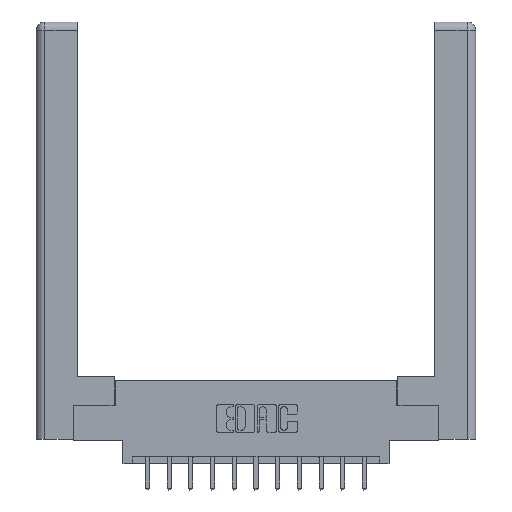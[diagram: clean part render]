
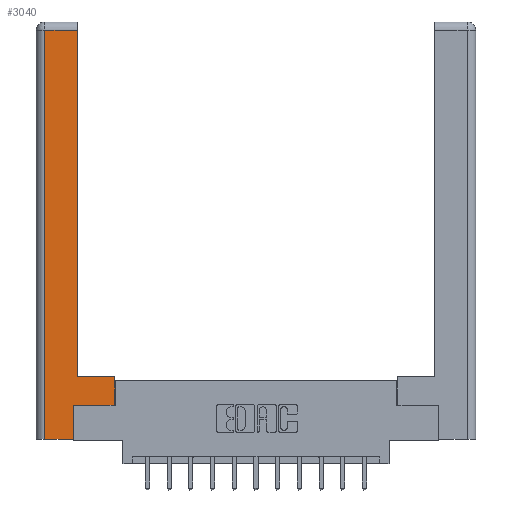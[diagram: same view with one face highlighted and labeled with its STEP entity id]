
A CAD part, top view. The second image highlights one B-rep face of the part: STEP entity #3040.
In plain terms, the highlighted planar face has unit normal (0, 0, 1).
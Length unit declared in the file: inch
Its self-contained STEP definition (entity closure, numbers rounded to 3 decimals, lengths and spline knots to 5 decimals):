
#283 = CARTESIAN_POINT ( 'NONE',  ( 0.265, 0., 0. ) ) ;
#387 = CARTESIAN_POINT ( 'NONE',  ( 0.0615, 2.94, 0. ) ) ;
#875 = VERTEX_POINT ( 'NONE', #7731 ) ;
#1022 = FACE_OUTER_BOUND ( 'NONE', #5512, .T. ) ;
#1030 = LINE ( 'NONE', #3409, #8114 ) ;
#1248 = LINE ( 'NONE', #7853, #13894 ) ;
#1259 = LINE ( 'NONE', #15097, #13539 ) ;
#1558 = VERTEX_POINT ( 'NONE', #4169 ) ;
#1929 = ORIENTED_EDGE ( 'NONE', *, *, #6298, .T. ) ;
#2094 = ORIENTED_EDGE ( 'NONE', *, *, #11005, .T. ) ;
#2224 = VECTOR ( 'NONE', #11362, 39.37008 ) ;
#2547 = CARTESIAN_POINT ( 'NONE',  ( 0., 0., 0. ) ) ;
#2564 = DIRECTION ( 'NONE',  ( -1., 0., 0. ) ) ;
#2680 = DIRECTION ( 'NONE',  ( 1., 0., 0. ) ) ;
#3040 = ADVANCED_FACE ( 'NONE', ( #1022 ), #9620, .F. ) ;
#3053 = CARTESIAN_POINT ( 'NONE',  ( 0.0615, 0., 0. ) ) ;
#3153 = LINE ( 'NONE', #9420, #7616 ) ;
#3323 = CARTESIAN_POINT ( 'NONE',  ( 0.265, 0., 0. ) ) ;
#3409 = CARTESIAN_POINT ( 'NONE',  ( 0.295, 3., 0. ) ) ;
#3487 = VERTEX_POINT ( 'NONE', #3323 ) ;
#3609 = DIRECTION ( 'NONE',  ( 0., 0., -1. ) ) ;
#3932 = VERTEX_POINT ( 'NONE', #7294 ) ;
#4169 = CARTESIAN_POINT ( 'NONE',  ( 0.295, 0.45, 0. ) ) ;
#4195 = LINE ( 'NONE', #14065, #10153 ) ;
#4421 = LINE ( 'NONE', #7744, #9082 ) ;
#4822 = VERTEX_POINT ( 'NONE', #387 ) ;
#5071 = ORIENTED_EDGE ( 'NONE', *, *, #10920, .T. ) ;
#5512 = EDGE_LOOP ( 'NONE', ( #5071, #12639, #13416, #7903, #2094, #10251, #1929, #14564 ) ) ;
#5514 = CARTESIAN_POINT ( 'NONE',  ( 0.265, 0.245, 0. ) ) ;
#5577 = VERTEX_POINT ( 'NONE', #13350 ) ;
#5646 = VERTEX_POINT ( 'NONE', #7584 ) ;
#5843 = DIRECTION ( 'NONE',  ( 0., 1., 0. ) ) ;
#6298 = EDGE_CURVE ( 'NONE', #5577, #5646, #3153, .T. ) ;
#6750 = DIRECTION ( 'NONE',  ( -1., 0., 0. ) ) ;
#7294 = CARTESIAN_POINT ( 'NONE',  ( 0.0615, 0., 0. ) ) ;
#7584 = CARTESIAN_POINT ( 'NONE',  ( 0.565, 0.45, 0. ) ) ;
#7616 = VECTOR ( 'NONE', #5843, 39.37008 ) ;
#7731 = CARTESIAN_POINT ( 'NONE',  ( 0.295, 2.94, 0. ) ) ;
#7744 = CARTESIAN_POINT ( 'NONE',  ( 0.0615, 2.94, 0. ) ) ;
#7853 = CARTESIAN_POINT ( 'NONE',  ( 0.565, 0.245, 0. ) ) ;
#7903 = ORIENTED_EDGE ( 'NONE', *, *, #11271, .T. ) ;
#8114 = VECTOR ( 'NONE', #10632, 39.37008 ) ;
#8286 = DIRECTION ( 'NONE',  ( -1., 0., 0. ) ) ;
#8377 = LINE ( 'NONE', #3053, #2224 ) ;
#8821 = AXIS2_PLACEMENT_3D ( 'NONE', #2547, #3609, #8286 ) ;
#9082 = VECTOR ( 'NONE', #6750, 39.37008 ) ;
#9420 = CARTESIAN_POINT ( 'NONE',  ( 0.565, 0.45, 0. ) ) ;
#9620 = PLANE ( 'NONE',  #8821 ) ;
#9886 = EDGE_CURVE ( 'NONE', #875, #4822, #4421, .T. ) ;
#10153 = VECTOR ( 'NONE', #14480, 39.37008 ) ;
#10251 = ORIENTED_EDGE ( 'NONE', *, *, #15124, .T. ) ;
#10632 = DIRECTION ( 'NONE',  ( 0., 1., 0. ) ) ;
#10920 = EDGE_CURVE ( 'NONE', #1558, #875, #1030, .T. ) ;
#11005 = EDGE_CURVE ( 'NONE', #3487, #12149, #4195, .T. ) ;
#11271 = EDGE_CURVE ( 'NONE', #3932, #3487, #13492, .T. ) ;
#11362 = DIRECTION ( 'NONE',  ( 0., -1., 0. ) ) ;
#12019 = VECTOR ( 'NONE', #2680, 39.37008 ) ;
#12149 = VERTEX_POINT ( 'NONE', #5514 ) ;
#12616 = DIRECTION ( 'NONE',  ( 1., 0., 0. ) ) ;
#12639 = ORIENTED_EDGE ( 'NONE', *, *, #9886, .T. ) ;
#13042 = EDGE_CURVE ( 'NONE', #4822, #3932, #8377, .T. ) ;
#13350 = CARTESIAN_POINT ( 'NONE',  ( 0.565, 0.245, 0. ) ) ;
#13416 = ORIENTED_EDGE ( 'NONE', *, *, #13042, .T. ) ;
#13492 = LINE ( 'NONE', #283, #12019 ) ;
#13539 = VECTOR ( 'NONE', #2564, 39.37008 ) ;
#13894 = VECTOR ( 'NONE', #12616, 39.37008 ) ;
#14065 = CARTESIAN_POINT ( 'NONE',  ( 0.265, 0.245, 0. ) ) ;
#14480 = DIRECTION ( 'NONE',  ( 0., 1., 0. ) ) ;
#14564 = ORIENTED_EDGE ( 'NONE', *, *, #14925, .T. ) ;
#14925 = EDGE_CURVE ( 'NONE', #5646, #1558, #1259, .T. ) ;
#15097 = CARTESIAN_POINT ( 'NONE',  ( 0.295, 0.45, 0. ) ) ;
#15124 = EDGE_CURVE ( 'NONE', #12149, #5577, #1248, .T. ) ;
